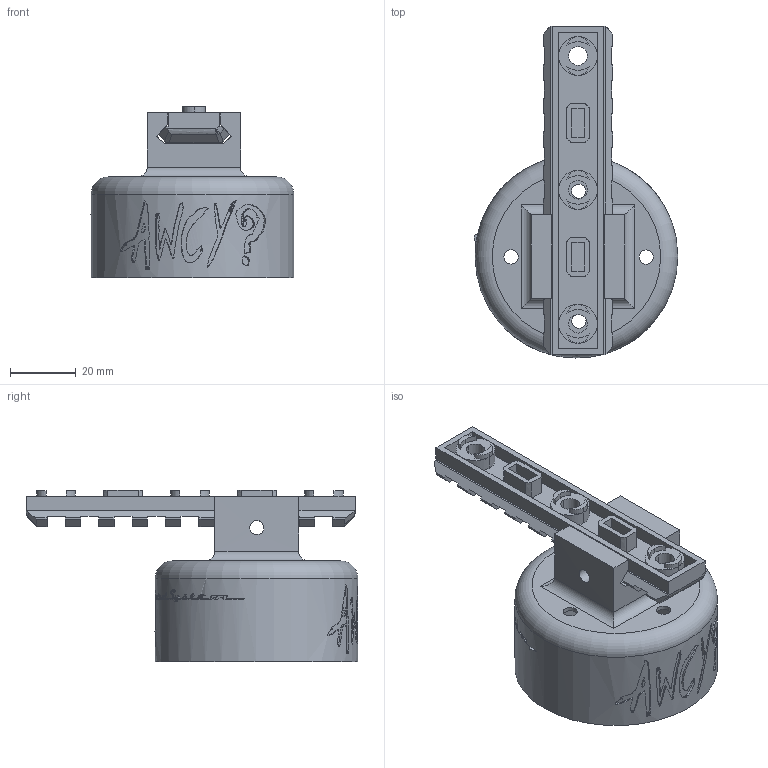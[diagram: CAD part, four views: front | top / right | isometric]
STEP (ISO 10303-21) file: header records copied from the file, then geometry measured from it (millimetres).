
FILE_DESCRIPTION(('STEP AP214'),'1');
FILE_NAME('HMB system- WC.stp','2021-01-18T20:15:36',(' '),(' '),'Spatial InterOp 3D',' ',' ');
FILE_SCHEMA(('AUTOMOTIVE_DESIGN { 1 0 10303 214 1 1 1 1 }'));
Length unit declared in the file: metre
Products named in the file (4): HMB system.2; Lid; HMB system- WC; PICATINNY RAIL
Assembly tree (3 placements, depth 3):
  HMB system- WC
    HMB system.2
      Lid
    PICATINNY RAIL
Bounding box: 61.78 x 100.67 x 52.08 mm (x, y, z)
Volume: 32984 mm3; surface area: 28588.7 mm2
Topology: 6 solids, 7 shells, 3728 faces, 8940 edges, 5079 vertices
Faces by surface type: plane 2476, bspline 914, cone 203, cylinder 134, torus 1
Full cylindrical faces by diameter (mm): 4.3 x5, 54.876 x1, 57.5 x1, 61.5 x1
Entity records: 153444 total; most frequent: CARTESIAN_POINT 66933, ORIENTED_EDGE 16992, DIRECTION 12644, EDGE_CURVE 8496, LINE 5862, VECTOR 5862, VERTEX_POINT 5011, EDGE_LOOP 3819
